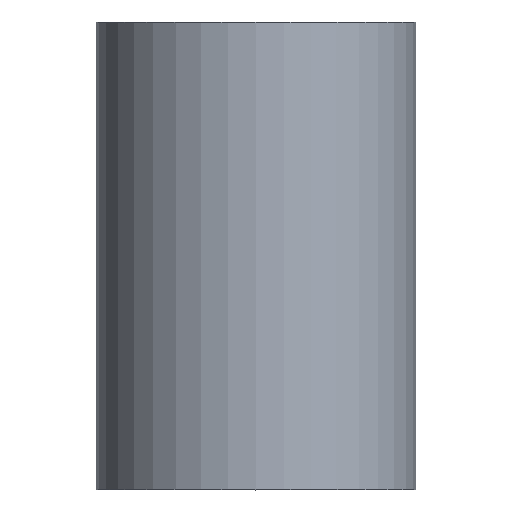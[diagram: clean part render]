
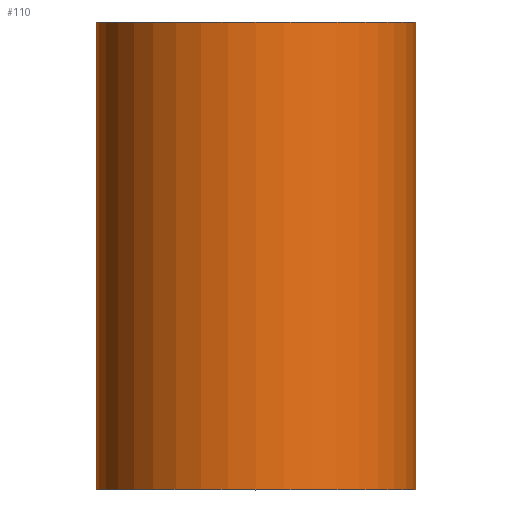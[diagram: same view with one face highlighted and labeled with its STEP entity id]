
A CAD part, top view. The second image highlights one B-rep face of the part: STEP entity #110.
In plain terms, the highlighted cylindrical face has radius 17.646 mm (diameter 35.292 mm), a full revolution.
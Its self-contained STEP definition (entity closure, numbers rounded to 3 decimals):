
#17=LINE('',#195,#21);
#21=VECTOR('',#160,17.646);
#25=CYLINDRICAL_SURFACE('',#135,17.646);
#34=FACE_OUTER_BOUND('',#43,.T.);
#43=EDGE_LOOP('',(#83,#84,#85,#86));
#53=CIRCLE('',#133,17.646);
#55=CIRCLE('',#136,17.646);
#61=VERTEX_POINT('',#188);
#63=VERTEX_POINT('',#193);
#69=EDGE_CURVE('',#61,#61,#53,.T.);
#71=EDGE_CURVE('',#63,#63,#55,.T.);
#72=EDGE_CURVE('',#63,#61,#17,.T.);
#83=ORIENTED_EDGE('',*,*,#71,.F.);
#84=ORIENTED_EDGE('',*,*,#72,.T.);
#85=ORIENTED_EDGE('',*,*,#69,.T.);
#86=ORIENTED_EDGE('',*,*,#72,.F.);
#110=ADVANCED_FACE('',(#34),#25,.T.);
#133=AXIS2_PLACEMENT_3D('',#189,#152,#153);
#135=AXIS2_PLACEMENT_3D('',#192,#156,#157);
#136=AXIS2_PLACEMENT_3D('',#194,#158,#159);
#152=DIRECTION('center_axis',(0.,-1.,0.));
#153=DIRECTION('ref_axis',(1.,0.,0.));
#156=DIRECTION('center_axis',(0.,-1.,0.));
#157=DIRECTION('ref_axis',(1.,0.,0.));
#158=DIRECTION('center_axis',(0.,-1.,0.));
#159=DIRECTION('ref_axis',(1.,0.,0.));
#160=DIRECTION('',(0.,1.,0.));
#188=CARTESIAN_POINT('',(-17.646,51.6,0.));
#189=CARTESIAN_POINT('Origin',(0.,51.6,0.));
#192=CARTESIAN_POINT('Origin',(0.,25.8,0.));
#193=CARTESIAN_POINT('',(-17.646,0.,0.));
#194=CARTESIAN_POINT('Origin',(0.,0.,0.));
#195=CARTESIAN_POINT('',(-17.646,25.8,0.));
